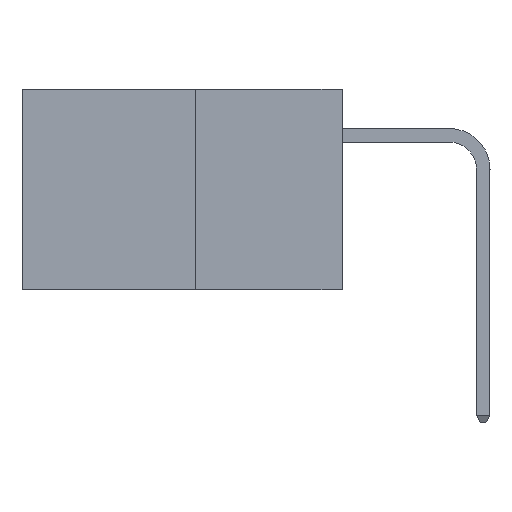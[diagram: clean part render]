
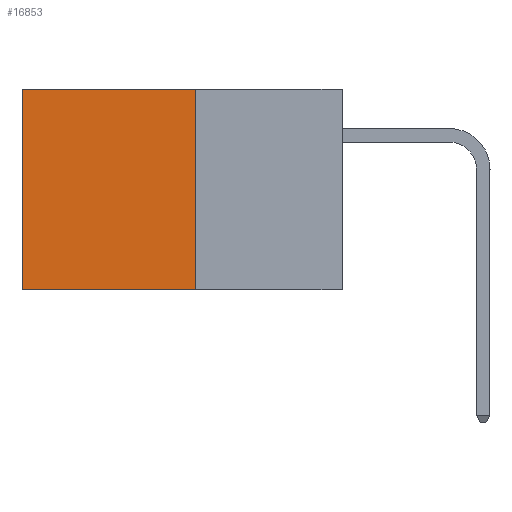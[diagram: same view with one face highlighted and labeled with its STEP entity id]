
A CAD part, left-side view. The second image highlights one B-rep face of the part: STEP entity #16853.
In plain terms, the highlighted planar face has unit normal (-1, 0, 0).
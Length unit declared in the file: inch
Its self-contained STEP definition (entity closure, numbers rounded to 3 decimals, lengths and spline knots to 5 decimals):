
#184 = CARTESIAN_POINT ( 'NONE',  ( 0.277, 0.59, -0.37 ) ) ;
#1054 = LINE ( 'NONE', #14578, #12170 ) ;
#1392 = LINE ( 'NONE', #10057, #17363 ) ;
#1597 = EDGE_CURVE ( 'NONE', #4053, #5066, #14004, .T. ) ;
#2019 = DIRECTION ( 'NONE',  ( 0., 0., -1. ) ) ;
#2101 = EDGE_CURVE ( 'NONE', #4053, #8547, #1054, .T. ) ;
#2348 = CARTESIAN_POINT ( 'NONE',  ( 0.277, 0.59, -0.37 ) ) ;
#2548 = ORIENTED_EDGE ( 'NONE', *, *, #15461, .F. ) ;
#3003 = ORIENTED_EDGE ( 'NONE', *, *, #1597, .T. ) ;
#4053 = VERTEX_POINT ( 'NONE', #8046 ) ;
#4311 = CARTESIAN_POINT ( 'NONE',  ( 0.277, 0.59, 0. ) ) ;
#4364 = PLANE ( 'NONE',  #17864 ) ;
#5066 = VERTEX_POINT ( 'NONE', #4311 ) ;
#5904 = DIRECTION ( 'NONE',  ( 0., 0., -1. ) ) ;
#6581 = ORIENTED_EDGE ( 'NONE', *, *, #2101, .F. ) ;
#8046 = CARTESIAN_POINT ( 'NONE',  ( 0.277, 0.27, 0. ) ) ;
#8547 = VERTEX_POINT ( 'NONE', #12795 ) ;
#8756 = EDGE_LOOP ( 'NONE', ( #14084, #2548, #6581, #3003 ) ) ;
#9250 = LINE ( 'NONE', #2348, #16704 ) ;
#9802 = EDGE_CURVE ( 'NONE', #5066, #12115, #9250, .T. ) ;
#10057 = CARTESIAN_POINT ( 'NONE',  ( 0.277, 0.27, -0.37 ) ) ;
#10399 = CARTESIAN_POINT ( 'NONE',  ( 0.277, 0.27, -0.37 ) ) ;
#11250 = CARTESIAN_POINT ( 'NONE',  ( 0.277, 0.27, 0. ) ) ;
#11251 = DIRECTION ( 'NONE',  ( 0., 1., 0. ) ) ;
#11916 = DIRECTION ( 'NONE',  ( 0., 0., -1. ) ) ;
#12115 = VERTEX_POINT ( 'NONE', #184 ) ;
#12170 = VECTOR ( 'NONE', #11916, 39.37008 ) ;
#12795 = CARTESIAN_POINT ( 'NONE',  ( 0.277, 0.27, -0.37 ) ) ;
#14004 = LINE ( 'NONE', #11250, #17496 ) ;
#14042 = FACE_OUTER_BOUND ( 'NONE', #8756, .T. ) ;
#14084 = ORIENTED_EDGE ( 'NONE', *, *, #9802, .T. ) ;
#14578 = CARTESIAN_POINT ( 'NONE',  ( 0.277, 0.27, -0.37 ) ) ;
#14889 = DIRECTION ( 'NONE',  ( 1., 0., 0. ) ) ;
#15461 = EDGE_CURVE ( 'NONE', #8547, #12115, #1392, .T. ) ;
#16033 = DIRECTION ( 'NONE',  ( 0., 1., 0. ) ) ;
#16704 = VECTOR ( 'NONE', #2019, 39.37008 ) ;
#16853 = ADVANCED_FACE ( 'NONE', ( #14042 ), #4364, .F. ) ;
#17363 = VECTOR ( 'NONE', #16033, 39.37008 ) ;
#17496 = VECTOR ( 'NONE', #11251, 39.37008 ) ;
#17864 = AXIS2_PLACEMENT_3D ( 'NONE', #10399, #14889, #5904 ) ;
